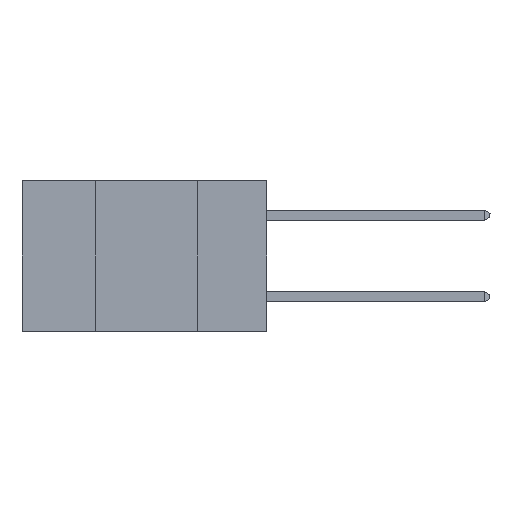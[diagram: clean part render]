
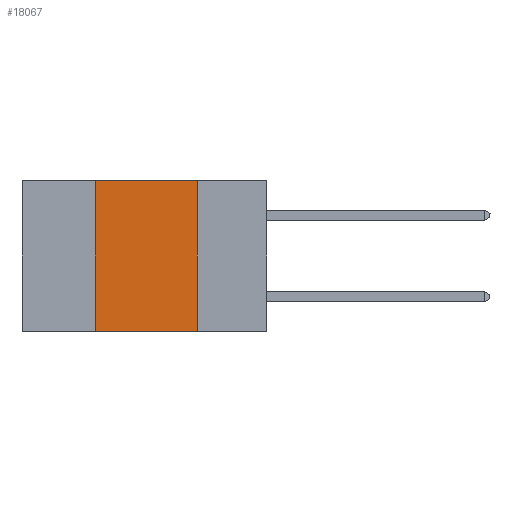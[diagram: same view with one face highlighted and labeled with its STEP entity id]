
A CAD part, left-side view. The second image highlights one B-rep face of the part: STEP entity #18067.
In plain terms, the highlighted planar face has unit normal (-1, 0, 0).
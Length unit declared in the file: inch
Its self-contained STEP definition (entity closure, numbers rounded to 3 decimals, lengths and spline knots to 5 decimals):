
#1120 = DIRECTION ( 'NONE',  ( 1., 0., 0. ) ) ;
#1566 = VECTOR ( 'NONE', #22243, 39.37008 ) ;
#2582 = CARTESIAN_POINT ( 'NONE',  ( 0., 0.17, 0. ) ) ;
#3882 = DIRECTION ( 'NONE',  ( 0., -1., 0. ) ) ;
#4810 = PLANE ( 'NONE',  #10731 ) ;
#5503 = VERTEX_POINT ( 'NONE', #9807 ) ;
#6020 = EDGE_CURVE ( 'NONE', #18557, #5503, #10145, .T. ) ;
#6187 = DIRECTION ( 'NONE',  ( 0., 0., -1. ) ) ;
#6425 = ORIENTED_EDGE ( 'NONE', *, *, #15051, .F. ) ;
#6665 = LINE ( 'NONE', #8768, #18283 ) ;
#7270 = ORIENTED_EDGE ( 'NONE', *, *, #19646, .F. ) ;
#8768 = CARTESIAN_POINT ( 'NONE',  ( 0., 0.6, 0. ) ) ;
#9778 = EDGE_LOOP ( 'NONE', ( #16126, #7270, #6425, #19390 ) ) ;
#9807 = CARTESIAN_POINT ( 'NONE',  ( 0., 0.17, -0.37 ) ) ;
#10026 = CARTESIAN_POINT ( 'NONE',  ( 0., 0.17, 0. ) ) ;
#10047 = VERTEX_POINT ( 'NONE', #19125 ) ;
#10145 = LINE ( 'NONE', #10026, #12776 ) ;
#10731 = AXIS2_PLACEMENT_3D ( 'NONE', #12606, #1120, #12363 ) ;
#11002 = EDGE_CURVE ( 'NONE', #14173, #5503, #20829, .T. ) ;
#11100 = CARTESIAN_POINT ( 'NONE',  ( 0., 0.42, 0. ) ) ;
#12363 = DIRECTION ( 'NONE',  ( 0., 0., -1. ) ) ;
#12606 = CARTESIAN_POINT ( 'NONE',  ( 0., 0.6, 0. ) ) ;
#12776 = VECTOR ( 'NONE', #6187, 39.37008 ) ;
#14173 = VERTEX_POINT ( 'NONE', #16728 ) ;
#14214 = FACE_OUTER_BOUND ( 'NONE', #9778, .T. ) ;
#15051 = EDGE_CURVE ( 'NONE', #14173, #10047, #22120, .T. ) ;
#16126 = ORIENTED_EDGE ( 'NONE', *, *, #6020, .F. ) ;
#16728 = CARTESIAN_POINT ( 'NONE',  ( 0., 0.42, -0.37 ) ) ;
#18067 = ADVANCED_FACE ( 'NONE', ( #14214 ), #4810, .F. ) ;
#18283 = VECTOR ( 'NONE', #23522, 39.37008 ) ;
#18557 = VERTEX_POINT ( 'NONE', #2582 ) ;
#19125 = CARTESIAN_POINT ( 'NONE',  ( 0., 0.42, 0. ) ) ;
#19390 = ORIENTED_EDGE ( 'NONE', *, *, #11002, .T. ) ;
#19646 = EDGE_CURVE ( 'NONE', #10047, #18557, #6665, .T. ) ;
#20829 = LINE ( 'NONE', #21080, #21648 ) ;
#21080 = CARTESIAN_POINT ( 'NONE',  ( 0., 0.6, -0.37 ) ) ;
#21648 = VECTOR ( 'NONE', #3882, 39.37008 ) ;
#22120 = LINE ( 'NONE', #11100, #1566 ) ;
#22243 = DIRECTION ( 'NONE',  ( 0., 0., 1. ) ) ;
#23522 = DIRECTION ( 'NONE',  ( 0., -1., 0. ) ) ;
